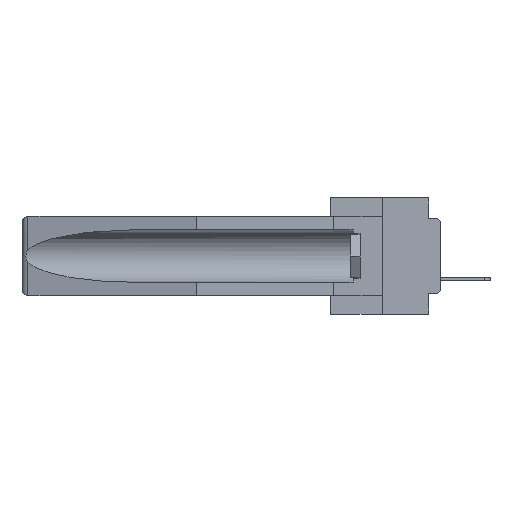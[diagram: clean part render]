
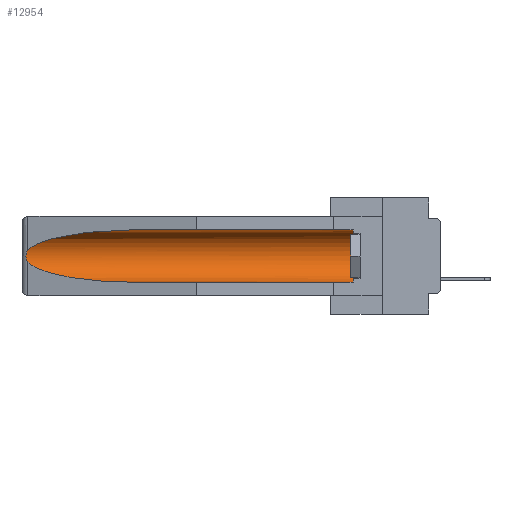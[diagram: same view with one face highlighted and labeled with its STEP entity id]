
A CAD part, left-side view. The second image highlights one B-rep face of the part: STEP entity #12954.
In plain terms, the highlighted cylindrical face has radius 2.857 mm (diameter 5.715 mm), a partial arc.
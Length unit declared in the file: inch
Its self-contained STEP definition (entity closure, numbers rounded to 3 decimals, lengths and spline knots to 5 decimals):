
#67 = CARTESIAN_POINT ( 'NONE',  ( 0.155, 1.07973, -0.284 ) ) ;
#289 = CARTESIAN_POINT ( 'NONE',  ( 0.26655, 1.53094, -0.18657 ) ) ;
#1633 = VECTOR ( 'NONE', #9003, 39.37008 ) ;
#3438 = DIRECTION ( 'NONE',  ( 0., 0., 1. ) ) ;
#4672 = EDGE_CURVE ( 'NONE', #26889, #21821, #14499, .T. ) ;
#5244 = CARTESIAN_POINT ( 'NONE',  ( 0.25451, 1.48313, -0.09465 ) ) ;
#5283 = DIRECTION ( 'NONE',  ( 0., 1., 0. ) ) ;
#5768 = CARTESIAN_POINT ( 'NONE',  ( 0.26537, 1.52718, -0.14972 ) ) ;
#5877 = EDGE_LOOP ( 'NONE', ( #18919, #13494, #26379, #25711, #17274, #21694 ) ) ;
#6254 =( BOUNDED_CURVE ( )  B_SPLINE_CURVE ( 3, ( #10936, #21443, #5244, #5768 ),
 .UNSPECIFIED., .F., .F. ) 
 B_SPLINE_CURVE_WITH_KNOTS ( ( 4, 4 ),
 ( 4.71239, 6.08839 ),
 .UNSPECIFIED. ) 
 CURVE ( )  GEOMETRIC_REPRESENTATION_ITEM ( )  RATIONAL_B_SPLINE_CURVE ( ( 1., 0.848, 0.848, 1. ) ) 
 REPRESENTATION_ITEM ( '' )  );
#6955 = VERTEX_POINT ( 'NONE', #31591 ) ;
#7235 = EDGE_CURVE ( 'NONE', #6955, #24789, #22614, .T. ) ;
#8006 = CIRCLE ( 'NONE', #24526, 0.1125 ) ;
#8057 = EDGE_CURVE ( 'NONE', #19734, #11079, #16492, .T. ) ;
#8221 = DIRECTION ( 'NONE',  ( 0., 0., 1. ) ) ;
#8407 = CARTESIAN_POINT ( 'NONE',  ( 0.26537, 1.52718, -0.14972 ) ) ;
#8585 = CARTESIAN_POINT ( 'NONE',  ( 0.2673, 1.5327, -0.16383 ) ) ;
#8832 = CARTESIAN_POINT ( 'NONE',  ( 0.155, -0.30754, -0.059 ) ) ;
#9003 = DIRECTION ( 'NONE',  ( 0., 1., 0. ) ) ;
#9594 = EDGE_CURVE ( 'NONE', #11079, #24789, #21362, .T. ) ;
#9877 = DIRECTION ( 'NONE',  ( 0., 1., 0. ) ) ;
#10526 = CARTESIAN_POINT ( 'NONE',  ( 0.155, 0.126, -0.059 ) ) ;
#10936 = CARTESIAN_POINT ( 'NONE',  ( 0.155, 1.07973, -0.059 ) ) ;
#11079 = VERTEX_POINT ( 'NONE', #26661 ) ;
#11949 = CARTESIAN_POINT ( 'NONE',  ( 0.26537, 1.52718, -0.14972 ) ) ;
#12123 = CARTESIAN_POINT ( 'NONE',  ( 0.155, -0.30754, -0.284 ) ) ;
#12579 = CARTESIAN_POINT ( 'NONE',  ( 0.26537, 1.52718, -0.19328 ) ) ;
#12954 = ADVANCED_FACE ( 'NONE', ( #13237 ), #15984, .F. ) ;
#13237 = FACE_OUTER_BOUND ( 'NONE', #5877, .T. ) ;
#13494 = ORIENTED_EDGE ( 'NONE', *, *, #8057, .T. ) ;
#14499 = LINE ( 'NONE', #8832, #1633 ) ;
#15984 = CYLINDRICAL_SURFACE ( 'NONE', #28390, 0.1125 ) ;
#16492 = B_SPLINE_CURVE_WITH_KNOTS ( 'NONE', 3,
 ( #8407, #21671, #32165, #8585, #26992, #21846, #32342, #289, #18922, #31988 ),
 .UNSPECIFIED., .F., .F.,
 ( 4, 2, 2, 2, 4 ),
 ( 0., 0.00029, 0.00058, 0.00087, 0.00117 ),
 .UNSPECIFIED. ) ;
#17274 = ORIENTED_EDGE ( 'NONE', *, *, #24544, .T. ) ;
#18919 = ORIENTED_EDGE ( 'NONE', *, *, #29998, .T. ) ;
#18922 = CARTESIAN_POINT ( 'NONE',  ( 0.26597, 1.5296, -0.19026 ) ) ;
#19734 = VERTEX_POINT ( 'NONE', #11949 ) ;
#20154 = CARTESIAN_POINT ( 'NONE',  ( 0.21114, 1.30732, -0.284 ) ) ;
#20317 = CARTESIAN_POINT ( 'NONE',  ( 0.25451, 1.48313, -0.24835 ) ) ;
#21362 =( BOUNDED_CURVE ( )  B_SPLINE_CURVE ( 3, ( #12579, #20317, #20154, #23057 ),
 .UNSPECIFIED., .F., .F. ) 
 B_SPLINE_CURVE_WITH_KNOTS ( ( 4, 4 ),
 ( 0.1948, 1.5708 ),
 .UNSPECIFIED. ) 
 CURVE ( )  GEOMETRIC_REPRESENTATION_ITEM ( )  RATIONAL_B_SPLINE_CURVE ( ( 1., 0.848, 0.848, 1. ) ) 
 REPRESENTATION_ITEM ( '' )  );
#21443 = CARTESIAN_POINT ( 'NONE',  ( 0.21114, 1.30732, -0.059 ) ) ;
#21531 = CARTESIAN_POINT ( 'NONE',  ( 0.155, 0.126, -0.1715 ) ) ;
#21671 = CARTESIAN_POINT ( 'NONE',  ( 0.26597, 1.52961, -0.15275 ) ) ;
#21694 = ORIENTED_EDGE ( 'NONE', *, *, #4672, .T. ) ;
#21821 = VERTEX_POINT ( 'NONE', #27049 ) ;
#21846 = CARTESIAN_POINT ( 'NONE',  ( 0.2675, 1.53308, -0.17534 ) ) ;
#22614 = LINE ( 'NONE', #12123, #30390 ) ;
#23057 = CARTESIAN_POINT ( 'NONE',  ( 0.155, 1.07973, -0.284 ) ) ;
#24526 = AXIS2_PLACEMENT_3D ( 'NONE', #21531, #29623, #3438 ) ;
#24544 = EDGE_CURVE ( 'NONE', #6955, #26889, #8006, .T. ) ;
#24789 = VERTEX_POINT ( 'NONE', #67 ) ;
#25711 = ORIENTED_EDGE ( 'NONE', *, *, #7235, .F. ) ;
#26379 = ORIENTED_EDGE ( 'NONE', *, *, #9594, .T. ) ;
#26661 = CARTESIAN_POINT ( 'NONE',  ( 0.26537, 1.52718, -0.19328 ) ) ;
#26889 = VERTEX_POINT ( 'NONE', #10526 ) ;
#26992 = CARTESIAN_POINT ( 'NONE',  ( 0.2675, 1.53308, -0.16763 ) ) ;
#27049 = CARTESIAN_POINT ( 'NONE',  ( 0.155, 1.07973, -0.059 ) ) ;
#28390 = AXIS2_PLACEMENT_3D ( 'NONE', #29580, #5283, #8221 ) ;
#29580 = CARTESIAN_POINT ( 'NONE',  ( 0.155, -0.30754, -0.1715 ) ) ;
#29623 = DIRECTION ( 'NONE',  ( 0., -1., 0. ) ) ;
#29998 = EDGE_CURVE ( 'NONE', #21821, #19734, #6254, .T. ) ;
#30390 = VECTOR ( 'NONE', #9877, 39.37008 ) ;
#31591 = CARTESIAN_POINT ( 'NONE',  ( 0.155, 0.126, -0.284 ) ) ;
#31988 = CARTESIAN_POINT ( 'NONE',  ( 0.26537, 1.52718, -0.19328 ) ) ;
#32165 = CARTESIAN_POINT ( 'NONE',  ( 0.26654, 1.53092, -0.15636 ) ) ;
#32342 = CARTESIAN_POINT ( 'NONE',  ( 0.2673, 1.53269, -0.17917 ) ) ;
